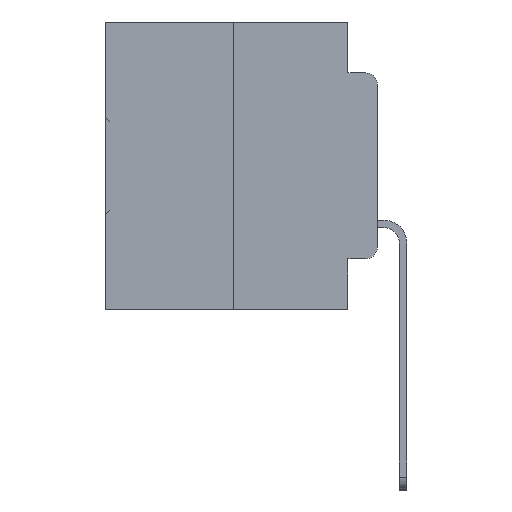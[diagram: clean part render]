
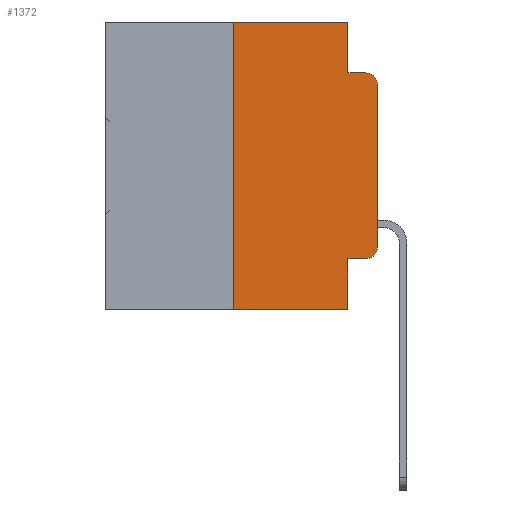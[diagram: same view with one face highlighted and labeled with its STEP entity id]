
A CAD part, left-side view. The second image highlights one B-rep face of the part: STEP entity #1372.
In plain terms, the highlighted planar face has unit normal (-1, 0, 0).
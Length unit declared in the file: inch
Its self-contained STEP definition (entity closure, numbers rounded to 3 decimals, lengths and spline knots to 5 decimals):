
#499 = EDGE_CURVE ( 'NONE', #1497, #15945, #9362, .T. ) ;
#561 = AXIS2_PLACEMENT_3D ( 'NONE', #18285, #2111, #21033 ) ;
#883 = DIRECTION ( 'NONE',  ( 0., -1., 0. ) ) ;
#1145 = DIRECTION ( 'NONE',  ( 1., 0., 0. ) ) ;
#1372 = ADVANCED_FACE ( 'NONE', ( #21139 ), #12382, .F. ) ;
#1497 = VERTEX_POINT ( 'NONE', #14872 ) ;
#1590 = AXIS2_PLACEMENT_3D ( 'NONE', #9564, #28435, #12289 ) ;
#2111 = DIRECTION ( 'NONE',  ( -1., 0., 0. ) ) ;
#3232 = VERTEX_POINT ( 'NONE', #16565 ) ;
#3374 = CARTESIAN_POINT ( 'NONE',  ( 0., 0.051, -0.5 ) ) ;
#3961 = EDGE_LOOP ( 'NONE', ( #31691, #25007, #32994, #14953, #28923, #8672, #22663, #23104, #30666, #30739 ) ) ;
#4112 = DIRECTION ( 'NONE',  ( 0., 0., -1. ) ) ;
#4456 = VECTOR ( 'NONE', #18802, 39.37008 ) ;
#4761 = EDGE_CURVE ( 'NONE', #32276, #30677, #29997, .T. ) ;
#5111 = CARTESIAN_POINT ( 'NONE',  ( 0., 0.473, 0. ) ) ;
#5341 = EDGE_CURVE ( 'NONE', #28059, #32276, #33708, .T. ) ;
#5885 = VECTOR ( 'NONE', #10934, 39.37008 ) ;
#6204 = CARTESIAN_POINT ( 'NONE',  ( 0., 0.051, -0.4115 ) ) ;
#6318 = AXIS2_PLACEMENT_3D ( 'NONE', #24518, #1145, #4112 ) ;
#6398 = EDGE_CURVE ( 'NONE', #30677, #1497, #28250, .T. ) ;
#7492 = VECTOR ( 'NONE', #27305, 39.37008 ) ;
#8672 = ORIENTED_EDGE ( 'NONE', *, *, #5341, .F. ) ;
#9362 = LINE ( 'NONE', #19206, #30044 ) ;
#9564 = CARTESIAN_POINT ( 'NONE',  ( 0., 0.02, -0.3915 ) ) ;
#9594 = VECTOR ( 'NONE', #883, 39.37008 ) ;
#9914 = VERTEX_POINT ( 'NONE', #14355 ) ;
#10934 = DIRECTION ( 'NONE',  ( 0., 0., 1. ) ) ;
#11120 = EDGE_CURVE ( 'NONE', #28059, #12454, #21880, .T. ) ;
#11307 = DIRECTION ( 'NONE',  ( 0., -1., 0. ) ) ;
#11969 = CARTESIAN_POINT ( 'NONE',  ( 0., 0.051, 0. ) ) ;
#12289 = DIRECTION ( 'NONE',  ( 0., 0., -1. ) ) ;
#12382 = PLANE ( 'NONE',  #6318 ) ;
#12454 = VERTEX_POINT ( 'NONE', #3374 ) ;
#12929 = EDGE_CURVE ( 'NONE', #3232, #33876, #18794, .T. ) ;
#13579 = CARTESIAN_POINT ( 'NONE',  ( 0., 0.02, -0.4115 ) ) ;
#14355 = CARTESIAN_POINT ( 'NONE',  ( 0., 0.051, -0.4115 ) ) ;
#14753 = VECTOR ( 'NONE', #26410, 39.37008 ) ;
#14848 = LINE ( 'NONE', #11969, #21206 ) ;
#14872 = CARTESIAN_POINT ( 'NONE',  ( 0., 0.051, -0.0885 ) ) ;
#14953 = ORIENTED_EDGE ( 'NONE', *, *, #6398, .F. ) ;
#15576 = CIRCLE ( 'NONE', #561, 0.02 ) ;
#15709 = CARTESIAN_POINT ( 'NONE',  ( 0., 0.051, 0. ) ) ;
#15945 = VERTEX_POINT ( 'NONE', #18366 ) ;
#16565 = CARTESIAN_POINT ( 'NONE',  ( 0., 0., -0.3915 ) ) ;
#16684 = EDGE_CURVE ( 'NONE', #28973, #3232, #25610, .T. ) ;
#17601 = CARTESIAN_POINT ( 'NONE',  ( 0., 0., -0.1085 ) ) ;
#17613 = LINE ( 'NONE', #6204, #9594 ) ;
#18285 = CARTESIAN_POINT ( 'NONE',  ( 0., 0.02, -0.1085 ) ) ;
#18366 = CARTESIAN_POINT ( 'NONE',  ( 0., 0.02, -0.0885 ) ) ;
#18794 = LINE ( 'NONE', #26823, #4456 ) ;
#18802 = DIRECTION ( 'NONE',  ( 0., 0., 1. ) ) ;
#19206 = CARTESIAN_POINT ( 'NONE',  ( 0., 0.051, -0.0885 ) ) ;
#20647 = EDGE_CURVE ( 'NONE', #33876, #15945, #15576, .T. ) ;
#21033 = DIRECTION ( 'NONE',  ( 0., 0., -1. ) ) ;
#21139 = FACE_OUTER_BOUND ( 'NONE', #3961, .T. ) ;
#21206 = VECTOR ( 'NONE', #33488, 39.37008 ) ;
#21880 = LINE ( 'NONE', #30014, #7492 ) ;
#22663 = ORIENTED_EDGE ( 'NONE', *, *, #11120, .T. ) ;
#23104 = ORIENTED_EDGE ( 'NONE', *, *, #30433, .F. ) ;
#23263 = CARTESIAN_POINT ( 'NONE',  ( 0., 0.25, 0. ) ) ;
#23720 = CARTESIAN_POINT ( 'NONE',  ( 0., 0.051, 0. ) ) ;
#24518 = CARTESIAN_POINT ( 'NONE',  ( 0., 0.473, 0. ) ) ;
#25007 = ORIENTED_EDGE ( 'NONE', *, *, #20647, .T. ) ;
#25610 = CIRCLE ( 'NONE', #1590, 0.02 ) ;
#26410 = DIRECTION ( 'NONE',  ( 0., 0., -1. ) ) ;
#26823 = CARTESIAN_POINT ( 'NONE',  ( 0., 0., 0. ) ) ;
#27305 = DIRECTION ( 'NONE',  ( 0., -1., 0. ) ) ;
#28059 = VERTEX_POINT ( 'NONE', #33520 ) ;
#28250 = LINE ( 'NONE', #23720, #14753 ) ;
#28435 = DIRECTION ( 'NONE',  ( -1., 0., 0. ) ) ;
#28923 = ORIENTED_EDGE ( 'NONE', *, *, #4761, .F. ) ;
#28973 = VERTEX_POINT ( 'NONE', #13579 ) ;
#29150 = VECTOR ( 'NONE', #30953, 39.37008 ) ;
#29776 = CARTESIAN_POINT ( 'NONE',  ( 0., 0.25, 0. ) ) ;
#29997 = LINE ( 'NONE', #5111, #29150 ) ;
#30014 = CARTESIAN_POINT ( 'NONE',  ( 0., 0.473, -0.5 ) ) ;
#30044 = VECTOR ( 'NONE', #11307, 39.37008 ) ;
#30433 = EDGE_CURVE ( 'NONE', #9914, #12454, #14848, .T. ) ;
#30666 = ORIENTED_EDGE ( 'NONE', *, *, #32685, .T. ) ;
#30677 = VERTEX_POINT ( 'NONE', #15709 ) ;
#30739 = ORIENTED_EDGE ( 'NONE', *, *, #16684, .T. ) ;
#30953 = DIRECTION ( 'NONE',  ( 0., -1., 0. ) ) ;
#31691 = ORIENTED_EDGE ( 'NONE', *, *, #12929, .T. ) ;
#32276 = VERTEX_POINT ( 'NONE', #23263 ) ;
#32685 = EDGE_CURVE ( 'NONE', #9914, #28973, #17613, .T. ) ;
#32994 = ORIENTED_EDGE ( 'NONE', *, *, #499, .F. ) ;
#33488 = DIRECTION ( 'NONE',  ( 0., 0., -1. ) ) ;
#33520 = CARTESIAN_POINT ( 'NONE',  ( 0., 0.25, -0.5 ) ) ;
#33708 = LINE ( 'NONE', #29776, #5885 ) ;
#33876 = VERTEX_POINT ( 'NONE', #17601 ) ;
